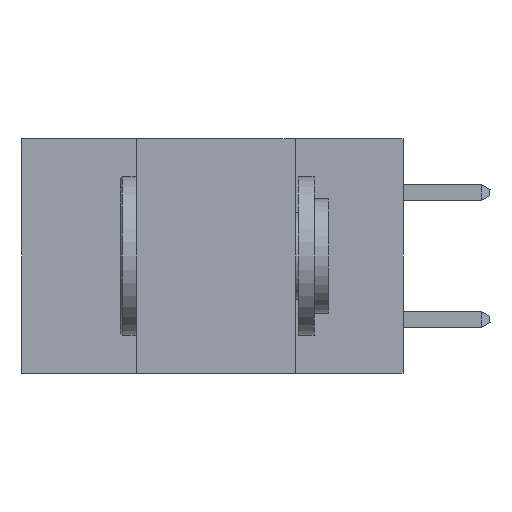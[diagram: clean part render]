
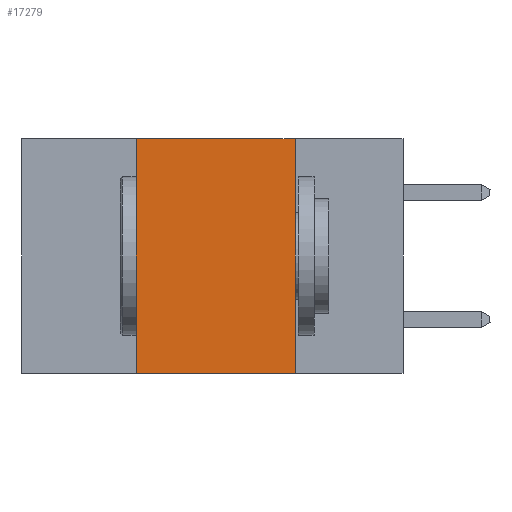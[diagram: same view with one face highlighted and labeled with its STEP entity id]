
A CAD part, left-side view. The second image highlights one B-rep face of the part: STEP entity #17279.
In plain terms, the highlighted planar face has unit normal (-1, 0, 0).
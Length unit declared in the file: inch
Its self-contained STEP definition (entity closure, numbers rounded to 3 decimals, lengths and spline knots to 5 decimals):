
#225 = EDGE_CURVE ( 'NONE', #30937, #31151, #22493, .T. ) ;
#2030 = CARTESIAN_POINT ( 'NONE',  ( 0., 0.42, 0. ) ) ;
#2255 = ORIENTED_EDGE ( 'NONE', *, *, #29641, .F. ) ;
#3503 = VERTEX_POINT ( 'NONE', #10049 ) ;
#4655 = FACE_OUTER_BOUND ( 'NONE', #32500, .T. ) ;
#4947 = EDGE_CURVE ( 'NONE', #31151, #8281, #8136, .T. ) ;
#7429 = DIRECTION ( 'NONE',  ( 0., 0., 1. ) ) ;
#8136 = LINE ( 'NONE', #18221, #16594 ) ;
#8281 = VERTEX_POINT ( 'NONE', #26348 ) ;
#8565 = CARTESIAN_POINT ( 'NONE',  ( 0., 0.42, 0. ) ) ;
#10049 = CARTESIAN_POINT ( 'NONE',  ( 0., 0.42, -0.37 ) ) ;
#10558 = LINE ( 'NONE', #2030, #29252 ) ;
#12095 = EDGE_CURVE ( 'NONE', #3503, #8281, #16498, .T. ) ;
#13131 = DIRECTION ( 'NONE',  ( 0., 0., -1. ) ) ;
#15583 = ORIENTED_EDGE ( 'NONE', *, *, #4947, .F. ) ;
#16498 = LINE ( 'NONE', #17818, #17334 ) ;
#16565 = ORIENTED_EDGE ( 'NONE', *, *, #12095, .T. ) ;
#16594 = VECTOR ( 'NONE', #13131, 39.37008 ) ;
#17279 = ADVANCED_FACE ( 'NONE', ( #4655 ), #22657, .F. ) ;
#17334 = VECTOR ( 'NONE', #33620, 39.37008 ) ;
#17818 = CARTESIAN_POINT ( 'NONE',  ( 0., 0.6, -0.37 ) ) ;
#18221 = CARTESIAN_POINT ( 'NONE',  ( 0., 0.17, 0. ) ) ;
#19206 = ORIENTED_EDGE ( 'NONE', *, *, #225, .F. ) ;
#19227 = VECTOR ( 'NONE', #29234, 39.37008 ) ;
#19331 = AXIS2_PLACEMENT_3D ( 'NONE', #24196, #22126, #21788 ) ;
#21154 = CARTESIAN_POINT ( 'NONE',  ( 0., 0.17, 0. ) ) ;
#21788 = DIRECTION ( 'NONE',  ( 0., 0., -1. ) ) ;
#22126 = DIRECTION ( 'NONE',  ( 1., 0., 0. ) ) ;
#22493 = LINE ( 'NONE', #31799, #19227 ) ;
#22657 = PLANE ( 'NONE',  #19331 ) ;
#24196 = CARTESIAN_POINT ( 'NONE',  ( 0., 0.6, 0. ) ) ;
#26348 = CARTESIAN_POINT ( 'NONE',  ( 0., 0.17, -0.37 ) ) ;
#29234 = DIRECTION ( 'NONE',  ( 0., -1., 0. ) ) ;
#29252 = VECTOR ( 'NONE', #7429, 39.37008 ) ;
#29641 = EDGE_CURVE ( 'NONE', #3503, #30937, #10558, .T. ) ;
#30937 = VERTEX_POINT ( 'NONE', #8565 ) ;
#31151 = VERTEX_POINT ( 'NONE', #21154 ) ;
#31799 = CARTESIAN_POINT ( 'NONE',  ( 0., 0.6, 0. ) ) ;
#32500 = EDGE_LOOP ( 'NONE', ( #15583, #19206, #2255, #16565 ) ) ;
#33620 = DIRECTION ( 'NONE',  ( 0., -1., 0. ) ) ;
